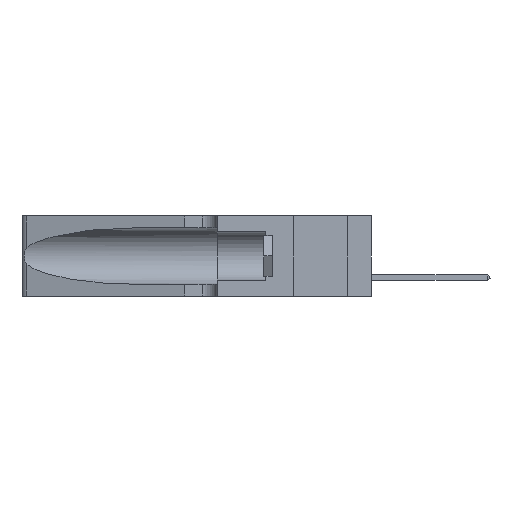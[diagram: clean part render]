
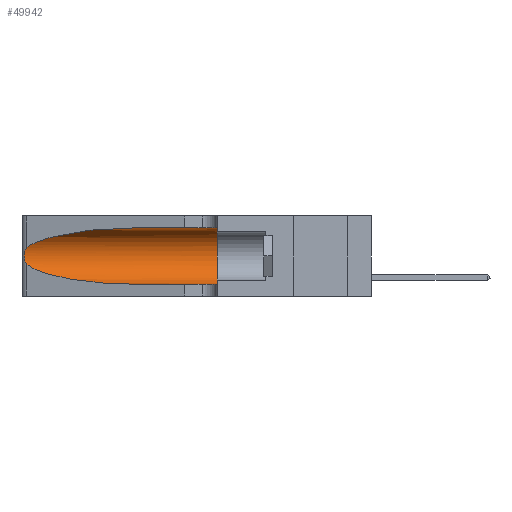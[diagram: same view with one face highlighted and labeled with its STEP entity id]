
A CAD part, left-side view. The second image highlights one B-rep face of the part: STEP entity #49942.
In plain terms, the highlighted cylindrical face has radius 3.308 mm (diameter 6.617 mm), a partial arc.
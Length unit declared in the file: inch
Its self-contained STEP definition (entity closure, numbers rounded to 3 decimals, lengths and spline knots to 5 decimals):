
#1420 = EDGE_CURVE ( 'NONE', #15008, #43970, #31104, .T. ) ;
#1749 = CARTESIAN_POINT ( 'NONE',  ( 0.2373, 1.15595, 0.08982 ) ) ;
#2313 = CARTESIAN_POINT ( 'NONE',  ( 0.1305, 1.61858, 0.05475 ) ) ;
#3462 = ORIENTED_EDGE ( 'NONE', *, *, #13697, .F. ) ;
#5064 = CARTESIAN_POINT ( 'NONE',  ( 0.1305, 1.61858, 0.185 ) ) ;
#5377 = ORIENTED_EDGE ( 'NONE', *, *, #12482, .T. ) ;
#5588 = CARTESIAN_POINT ( 'NONE',  ( 0.1305, 0.35, 0.05475 ) ) ;
#5878 = CARTESIAN_POINT ( 'NONE',  ( 0.25789, 1.23486, 0.15765 ) ) ;
#6259 = CARTESIAN_POINT ( 'NONE',  ( 0.25856, 1.23593, 0.16098 ) ) ;
#9493 = CARTESIAN_POINT ( 'NONE',  ( 0.1305, 0.72297, 0.31525 ) ) ;
#9768 = DIRECTION ( 'NONE',  ( 0., 0., 1. ) ) ;
#10058 = CARTESIAN_POINT ( 'NONE',  ( 0.25854, 1.2359, 0.20912 ) ) ;
#10386 = CARTESIAN_POINT ( 'NONE',  ( 0.1305, 1.61858, 0.31525 ) ) ;
#11812 = AXIS2_PLACEMENT_3D ( 'NONE', #33701, #29707, #9768 ) ;
#12482 = EDGE_CURVE ( 'NONE', #43970, #27624, #41830, .T. ) ;
#12948 = CARTESIAN_POINT ( 'NONE',  ( 0.25639, 1.23184, 0.21858 ) ) ;
#13697 = EDGE_CURVE ( 'NONE', #22833, #37114, #36609, .T. ) ;
#13846 = CARTESIAN_POINT ( 'NONE',  ( 0.25787, 1.23484, 0.2124 ) ) ;
#14245 = DIRECTION ( 'NONE',  ( 0., -1., 0. ) ) ;
#14351 = DIRECTION ( 'NONE',  ( 0., -1., 0. ) ) ;
#15008 = VERTEX_POINT ( 'NONE', #22644 ) ;
#16520 = CARTESIAN_POINT ( 'NONE',  ( 0.25487, 1.22718, 0.14631 ) ) ;
#17510 = DIRECTION ( 'NONE',  ( 0., 0., -1. ) ) ;
#18960 = ORIENTED_EDGE ( 'NONE', *, *, #36065, .T. ) ;
#19577 = EDGE_CURVE ( 'NONE', #37114, #40149, #22179, .T. ) ;
#20477 = VECTOR ( 'NONE', #14351, 39.37008 ) ;
#20643 = CARTESIAN_POINT ( 'NONE',  ( 0.1305, 0.72297, 0.31525 ) ) ;
#20962 = CARTESIAN_POINT ( 'NONE',  ( 0.1305, 0.35, 0.31525 ) ) ;
#21740 =( BOUNDED_CURVE ( )  B_SPLINE_CURVE ( 3, ( #20643, #45886, #33626, #37614 ),
 .UNSPECIFIED., .F., .T. ) 
 B_SPLINE_CURVE_WITH_KNOTS ( ( 4, 4 ),
 ( 1.5708, 2.84003 ),
 .UNSPECIFIED. ) 
 CURVE ( )  GEOMETRIC_REPRESENTATION_ITEM ( )  RATIONAL_B_SPLINE_CURVE ( ( 1., 0.87, 0.87, 1. ) ) 
 REPRESENTATION_ITEM ( '' )  );
#22179 = CIRCLE ( 'NONE', #11812, 0.13025 ) ;
#22644 = CARTESIAN_POINT ( 'NONE',  ( 0.25487, 1.22718, 0.22369 ) ) ;
#22833 = VERTEX_POINT ( 'NONE', #9493 ) ;
#23534 = ORIENTED_EDGE ( 'NONE', *, *, #19577, .F. ) ;
#26756 = CARTESIAN_POINT ( 'NONE',  ( 0.1305, 0.72297, 0.05475 ) ) ;
#27624 = VERTEX_POINT ( 'NONE', #26756 ) ;
#27723 = CYLINDRICAL_SURFACE ( 'NONE', #28097, 0.13025 ) ;
#27973 = CARTESIAN_POINT ( 'NONE',  ( 0.1305, 0.72297, 0.05475 ) ) ;
#28097 = AXIS2_PLACEMENT_3D ( 'NONE', #5064, #36602, #17510 ) ;
#28267 = FACE_OUTER_BOUND ( 'NONE', #42747, .T. ) ;
#29051 = LINE ( 'NONE', #2313, #47582 ) ;
#29607 = CARTESIAN_POINT ( 'NONE',  ( 0.26075, 1.23896, 0.19203 ) ) ;
#29707 = DIRECTION ( 'NONE',  ( 0., 1., 0. ) ) ;
#29809 = CARTESIAN_POINT ( 'NONE',  ( 0.26075, 1.23896, 0.178 ) ) ;
#31104 = B_SPLINE_CURVE_WITH_KNOTS ( 'NONE', 3,
 ( #37033, #37404, #12948, #13846, #10058, #49848, #29607, #29809, #41730, #6259, #5878, #38161, #34345, #42109 ),
 .UNSPECIFIED., .F., .F.,
 ( 4, 2, 2, 2, 2, 2, 4 ),
 ( 0., 0.00027, 0.00053, 0.00107, 0.0016, 0.00187, 0.00214 ),
 .UNSPECIFIED. ) ;
#32926 = ORIENTED_EDGE ( 'NONE', *, *, #1420, .T. ) ;
#33626 = CARTESIAN_POINT ( 'NONE',  ( 0.2373, 1.15595, 0.28018 ) ) ;
#33701 = CARTESIAN_POINT ( 'NONE',  ( 0.1305, 0.35, 0.185 ) ) ;
#34345 = CARTESIAN_POINT ( 'NONE',  ( 0.25555, 1.22993, 0.14849 ) ) ;
#36065 = EDGE_CURVE ( 'NONE', #27624, #40149, #29051, .T. ) ;
#36429 = ORIENTED_EDGE ( 'NONE', *, *, #36433, .T. ) ;
#36433 = EDGE_CURVE ( 'NONE', #22833, #15008, #21740, .T. ) ;
#36602 = DIRECTION ( 'NONE',  ( 0., -1., 0. ) ) ;
#36609 = LINE ( 'NONE', #10386, #20477 ) ;
#37033 = CARTESIAN_POINT ( 'NONE',  ( 0.25487, 1.22718, 0.22369 ) ) ;
#37114 = VERTEX_POINT ( 'NONE', #20962 ) ;
#37404 = CARTESIAN_POINT ( 'NONE',  ( 0.25555, 1.22994, 0.2215 ) ) ;
#37614 = CARTESIAN_POINT ( 'NONE',  ( 0.25487, 1.22718, 0.22369 ) ) ;
#38161 = CARTESIAN_POINT ( 'NONE',  ( 0.25639, 1.23186, 0.15144 ) ) ;
#40136 = CARTESIAN_POINT ( 'NONE',  ( 0.18966, 0.96281, 0.05475 ) ) ;
#40149 = VERTEX_POINT ( 'NONE', #5588 ) ;
#41456 = CARTESIAN_POINT ( 'NONE',  ( 0.25487, 1.22718, 0.14631 ) ) ;
#41730 = CARTESIAN_POINT ( 'NONE',  ( 0.26017, 1.23833, 0.17102 ) ) ;
#41830 =( BOUNDED_CURVE ( )  B_SPLINE_CURVE ( 3, ( #16520, #1749, #40136, #27973 ),
 .UNSPECIFIED., .F., .T. ) 
 B_SPLINE_CURVE_WITH_KNOTS ( ( 4, 4 ),
 ( 3.44316, 4.71239 ),
 .UNSPECIFIED. ) 
 CURVE ( )  GEOMETRIC_REPRESENTATION_ITEM ( )  RATIONAL_B_SPLINE_CURVE ( ( 1., 0.87, 0.87, 1. ) ) 
 REPRESENTATION_ITEM ( '' )  );
#42109 = CARTESIAN_POINT ( 'NONE',  ( 0.25487, 1.22718, 0.14631 ) ) ;
#42747 = EDGE_LOOP ( 'NONE', ( #36429, #32926, #5377, #18960, #23534, #3462 ) ) ;
#43970 = VERTEX_POINT ( 'NONE', #41456 ) ;
#45886 = CARTESIAN_POINT ( 'NONE',  ( 0.18966, 0.96281, 0.31525 ) ) ;
#47582 = VECTOR ( 'NONE', #14245, 39.37008 ) ;
#49848 = CARTESIAN_POINT ( 'NONE',  ( 0.26018, 1.23835, 0.19895 ) ) ;
#49942 = ADVANCED_FACE ( 'NONE', ( #28267 ), #27723, .F. ) ;
